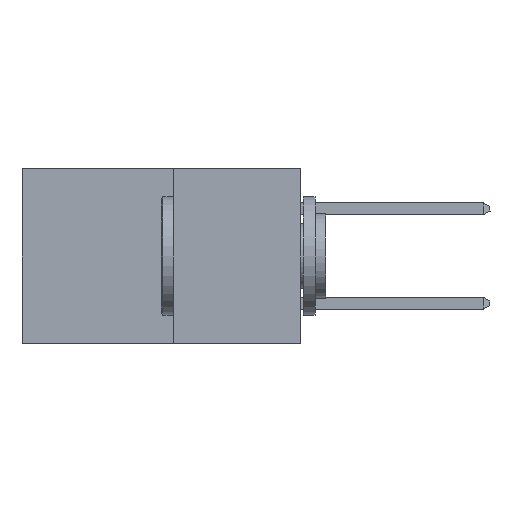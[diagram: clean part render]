
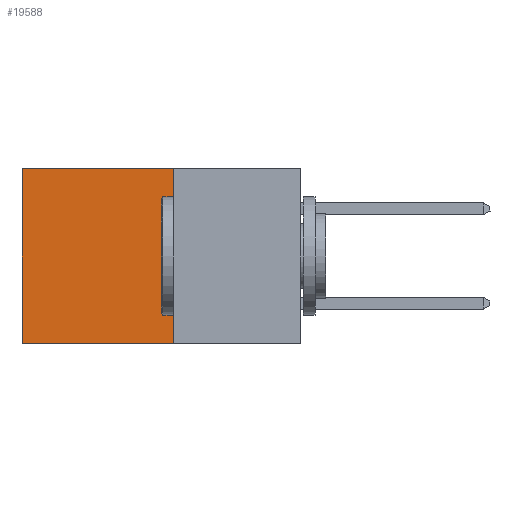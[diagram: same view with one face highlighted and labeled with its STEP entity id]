
A CAD part, left-side view. The second image highlights one B-rep face of the part: STEP entity #19588.
In plain terms, the highlighted planar face has unit normal (-1, 0, 0).
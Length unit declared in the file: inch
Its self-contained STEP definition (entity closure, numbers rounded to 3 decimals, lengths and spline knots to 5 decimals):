
#170 = VECTOR ( 'NONE', #6188, 39.37008 ) ;
#698 = LINE ( 'NONE', #1041, #6291 ) ;
#751 = DIRECTION ( 'NONE',  ( 0., 1., 0. ) ) ;
#922 = ORIENTED_EDGE ( 'NONE', *, *, #8904, .F. ) ;
#1041 = CARTESIAN_POINT ( 'NONE',  ( 0.277, 0.27, 0. ) ) ;
#1284 = CARTESIAN_POINT ( 'NONE',  ( 0.277, 0.27, -0.37 ) ) ;
#1660 = CARTESIAN_POINT ( 'NONE',  ( 0.277, 0.59, -0.37 ) ) ;
#1948 = CARTESIAN_POINT ( 'NONE',  ( 0.277, 0.59, -0.37 ) ) ;
#2399 = VECTOR ( 'NONE', #11829, 39.37008 ) ;
#2911 = AXIS2_PLACEMENT_3D ( 'NONE', #15426, #17493, #5152 ) ;
#3492 = EDGE_CURVE ( 'NONE', #16442, #10827, #16680, .T. ) ;
#3821 = EDGE_CURVE ( 'NONE', #16442, #15452, #698, .T. ) ;
#5152 = DIRECTION ( 'NONE',  ( 0., 0., -1. ) ) ;
#6188 = DIRECTION ( 'NONE',  ( 0., 0., -1. ) ) ;
#6291 = VECTOR ( 'NONE', #751, 39.37008 ) ;
#7295 = LINE ( 'NONE', #21965, #2399 ) ;
#7882 = FACE_OUTER_BOUND ( 'NONE', #10967, .T. ) ;
#8904 = EDGE_CURVE ( 'NONE', #10827, #12479, #7295, .T. ) ;
#9435 = ORIENTED_EDGE ( 'NONE', *, *, #3492, .F. ) ;
#10827 = VERTEX_POINT ( 'NONE', #1284 ) ;
#10967 = EDGE_LOOP ( 'NONE', ( #15113, #922, #9435, #17484 ) ) ;
#11829 = DIRECTION ( 'NONE',  ( 0., 1., 0. ) ) ;
#12479 = VERTEX_POINT ( 'NONE', #1948 ) ;
#13344 = PLANE ( 'NONE',  #2911 ) ;
#13519 = VECTOR ( 'NONE', #18173, 39.37008 ) ;
#15113 = ORIENTED_EDGE ( 'NONE', *, *, #22611, .T. ) ;
#15426 = CARTESIAN_POINT ( 'NONE',  ( 0.277, 0.27, -0.37 ) ) ;
#15452 = VERTEX_POINT ( 'NONE', #26090 ) ;
#16442 = VERTEX_POINT ( 'NONE', #20916 ) ;
#16680 = LINE ( 'NONE', #16944, #170 ) ;
#16944 = CARTESIAN_POINT ( 'NONE',  ( 0.277, 0.27, -0.37 ) ) ;
#17484 = ORIENTED_EDGE ( 'NONE', *, *, #3821, .T. ) ;
#17493 = DIRECTION ( 'NONE',  ( 1., 0., 0. ) ) ;
#18173 = DIRECTION ( 'NONE',  ( 0., 0., -1. ) ) ;
#18954 = LINE ( 'NONE', #1660, #13519 ) ;
#19588 = ADVANCED_FACE ( 'NONE', ( #7882 ), #13344, .F. ) ;
#20916 = CARTESIAN_POINT ( 'NONE',  ( 0.277, 0.27, 0. ) ) ;
#21965 = CARTESIAN_POINT ( 'NONE',  ( 0.277, 0.27, -0.37 ) ) ;
#22611 = EDGE_CURVE ( 'NONE', #15452, #12479, #18954, .T. ) ;
#26090 = CARTESIAN_POINT ( 'NONE',  ( 0.277, 0.59, 0. ) ) ;
